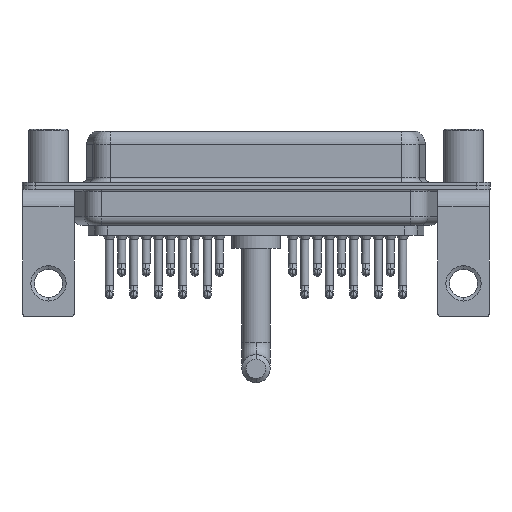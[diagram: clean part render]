
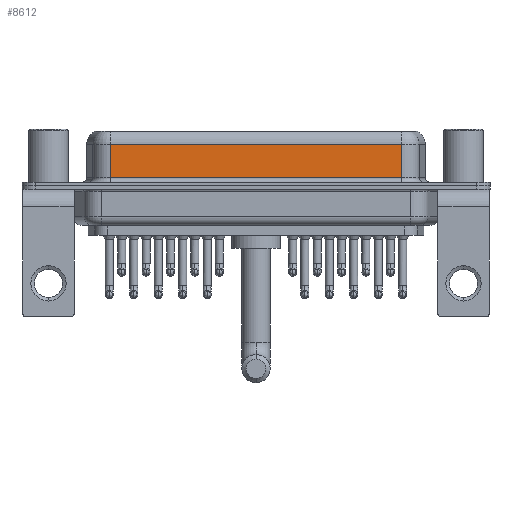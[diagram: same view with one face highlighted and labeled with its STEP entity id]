
A CAD part, front view. The second image highlights one B-rep face of the part: STEP entity #8612.
In plain terms, the highlighted planar face has unit normal (0, -1, 0).
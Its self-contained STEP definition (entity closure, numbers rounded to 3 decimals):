
#68 = PLANE ( 'NONE',  #23520 ) ;
#1003 = VECTOR ( 'NONE', #23138, 1000. ) ;
#1125 = CARTESIAN_POINT ( 'NONE',  ( 7.013, -3.95, 4.65 ) ) ;
#1538 = ORIENTED_EDGE ( 'NONE', *, *, #17537, .T. ) ;
#4050 = VERTEX_POINT ( 'NONE', #5242 ) ;
#4475 = EDGE_CURVE ( 'NONE', #10334, #4050, #25157, .T. ) ;
#5242 = CARTESIAN_POINT ( 'NONE',  ( 40.037, -3.95, 0.9 ) ) ;
#5512 = VECTOR ( 'NONE', #20884, 1000. ) ;
#5560 = CARTESIAN_POINT ( 'NONE',  ( 40.037, -3.95, 0.9 ) ) ;
#5810 = EDGE_CURVE ( 'NONE', #19906, #4050, #21591, .T. ) ;
#5812 = DIRECTION ( 'NONE',  ( 0., 0., 1. ) ) ;
#6086 = CARTESIAN_POINT ( 'NONE',  ( 40.037, -3.95, 4.65 ) ) ;
#6831 = CARTESIAN_POINT ( 'NONE',  ( 7.013, -3.95, 0.9 ) ) ;
#8229 = CARTESIAN_POINT ( 'NONE',  ( 40.037, -3.95, 6.4 ) ) ;
#8612 = ADVANCED_FACE ( 'NONE', ( #9879 ), #68, .F. ) ;
#9753 = DIRECTION ( 'NONE',  ( 0., 1., 0. ) ) ;
#9879 = FACE_OUTER_BOUND ( 'NONE', #13743, .T. ) ;
#10053 = CARTESIAN_POINT ( 'NONE',  ( 7.013, -3.95, 6.4 ) ) ;
#10334 = VERTEX_POINT ( 'NONE', #6831 ) ;
#11859 = VECTOR ( 'NONE', #13617, 1000. ) ;
#12030 = VECTOR ( 'NONE', #23761, 1000. ) ;
#13617 = DIRECTION ( 'NONE',  ( 0., 0., -1. ) ) ;
#13743 = EDGE_LOOP ( 'NONE', ( #18936, #14269, #1538, #15181 ) ) ;
#14269 = ORIENTED_EDGE ( 'NONE', *, *, #22744, .T. ) ;
#15181 = ORIENTED_EDGE ( 'NONE', *, *, #4475, .T. ) ;
#17523 = CARTESIAN_POINT ( 'NONE',  ( 40.037, -3.95, 6.4 ) ) ;
#17537 = EDGE_CURVE ( 'NONE', #17709, #10334, #18078, .T. ) ;
#17709 = VERTEX_POINT ( 'NONE', #1125 ) ;
#18078 = LINE ( 'NONE', #10053, #11859 ) ;
#18936 = ORIENTED_EDGE ( 'NONE', *, *, #5810, .F. ) ;
#18980 = CARTESIAN_POINT ( 'NONE',  ( 40.037, -3.95, 4.65 ) ) ;
#19906 = VERTEX_POINT ( 'NONE', #6086 ) ;
#20884 = DIRECTION ( 'NONE',  ( -1., 0., 0. ) ) ;
#21591 = LINE ( 'NONE', #8229, #12030 ) ;
#22744 = EDGE_CURVE ( 'NONE', #19906, #17709, #23184, .T. ) ;
#23138 = DIRECTION ( 'NONE',  ( 1., 0., 0. ) ) ;
#23184 = LINE ( 'NONE', #18980, #5512 ) ;
#23520 = AXIS2_PLACEMENT_3D ( 'NONE', #17523, #9753, #5812 ) ;
#23761 = DIRECTION ( 'NONE',  ( 0., 0., -1. ) ) ;
#25157 = LINE ( 'NONE', #5560, #1003 ) ;
